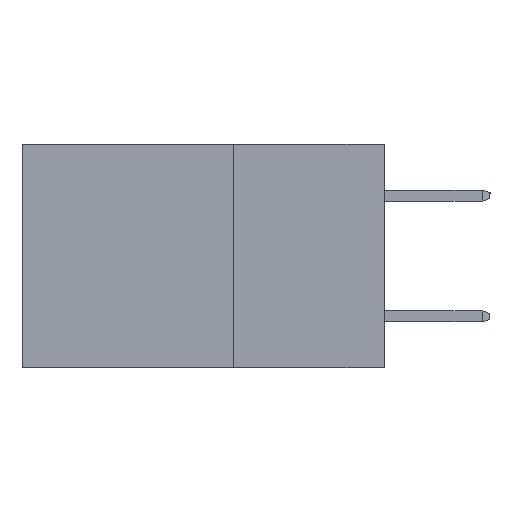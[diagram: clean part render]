
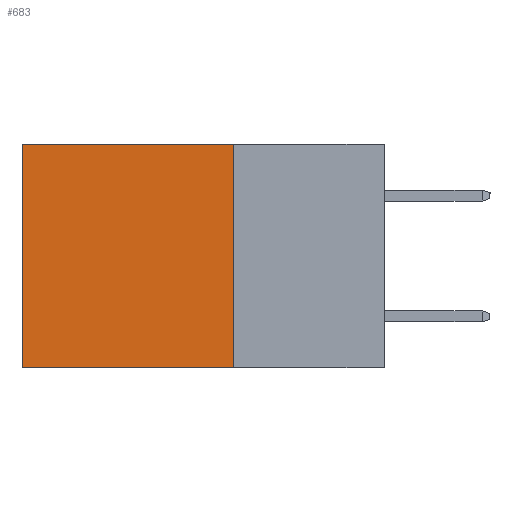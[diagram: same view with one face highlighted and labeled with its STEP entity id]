
A CAD part, left-side view. The second image highlights one B-rep face of the part: STEP entity #683.
In plain terms, the highlighted planar face has unit normal (-1, 0, 0).
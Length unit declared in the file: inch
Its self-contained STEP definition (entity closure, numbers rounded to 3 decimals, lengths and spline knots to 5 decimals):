
#189 = DIRECTION ( 'NONE',  ( 0., 1., 0. ) ) ;
#352 = CARTESIAN_POINT ( 'NONE',  ( 0.2615, 0.25, -0.37 ) ) ;
#683 = ADVANCED_FACE ( 'NONE', ( #1058 ), #1293, .F. ) ;
#697 = DIRECTION ( 'NONE',  ( 0., 0., -1. ) ) ;
#706 = EDGE_CURVE ( 'NONE', #8627, #7706, #2752, .T. ) ;
#1058 = FACE_OUTER_BOUND ( 'NONE', #7211, .T. ) ;
#1095 = VERTEX_POINT ( 'NONE', #8583 ) ;
#1119 = DIRECTION ( 'NONE',  ( 0., 0., -1. ) ) ;
#1293 = PLANE ( 'NONE',  #8293 ) ;
#1576 = EDGE_CURVE ( 'NONE', #8627, #1095, #7056, .T. ) ;
#1601 = CARTESIAN_POINT ( 'NONE',  ( 0.2615, 0.25, -0.37 ) ) ;
#1602 = CARTESIAN_POINT ( 'NONE',  ( 0.2615, 0.25, 0. ) ) ;
#1833 = VECTOR ( 'NONE', #697, 39.37008 ) ;
#2522 = ORIENTED_EDGE ( 'NONE', *, *, #706, .T. ) ;
#2740 = VECTOR ( 'NONE', #189, 39.37008 ) ;
#2752 = LINE ( 'NONE', #6515, #6256 ) ;
#2850 = CARTESIAN_POINT ( 'NONE',  ( 0.2615, 0.25, -0.37 ) ) ;
#3252 = LINE ( 'NONE', #1601, #2740 ) ;
#3519 = EDGE_CURVE ( 'NONE', #1095, #7145, #3252, .T. ) ;
#3897 = ORIENTED_EDGE ( 'NONE', *, *, #1576, .F. ) ;
#5239 = CARTESIAN_POINT ( 'NONE',  ( 0.2615, 0.6, -0.37 ) ) ;
#6256 = VECTOR ( 'NONE', #8738, 39.37008 ) ;
#6300 = VECTOR ( 'NONE', #1119, 39.37008 ) ;
#6502 = ORIENTED_EDGE ( 'NONE', *, *, #8129, .T. ) ;
#6515 = CARTESIAN_POINT ( 'NONE',  ( 0.2615, 0.25, 0. ) ) ;
#6962 = CARTESIAN_POINT ( 'NONE',  ( 0.2615, 0.6, 0. ) ) ;
#7056 = LINE ( 'NONE', #352, #6300 ) ;
#7091 = DIRECTION ( 'NONE',  ( 1., 0., 0. ) ) ;
#7145 = VERTEX_POINT ( 'NONE', #9175 ) ;
#7211 = EDGE_LOOP ( 'NONE', ( #6502, #8972, #3897, #2522 ) ) ;
#7264 = DIRECTION ( 'NONE',  ( 0., 0., -1. ) ) ;
#7500 = LINE ( 'NONE', #5239, #1833 ) ;
#7706 = VERTEX_POINT ( 'NONE', #6962 ) ;
#8129 = EDGE_CURVE ( 'NONE', #7706, #7145, #7500, .T. ) ;
#8293 = AXIS2_PLACEMENT_3D ( 'NONE', #2850, #7091, #7264 ) ;
#8583 = CARTESIAN_POINT ( 'NONE',  ( 0.2615, 0.25, -0.37 ) ) ;
#8627 = VERTEX_POINT ( 'NONE', #1602 ) ;
#8738 = DIRECTION ( 'NONE',  ( 0., 1., 0. ) ) ;
#8972 = ORIENTED_EDGE ( 'NONE', *, *, #3519, .F. ) ;
#9175 = CARTESIAN_POINT ( 'NONE',  ( 0.2615, 0.6, -0.37 ) ) ;
